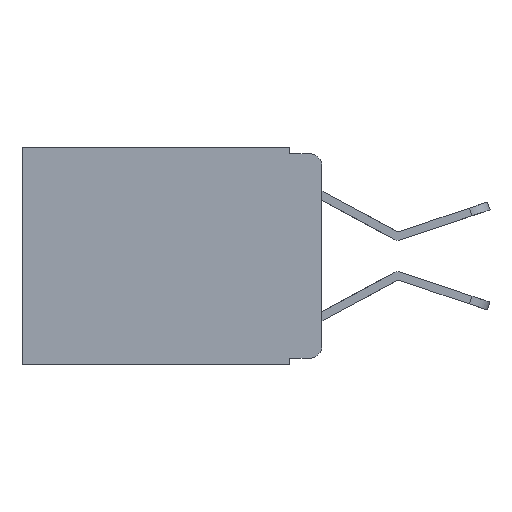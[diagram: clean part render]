
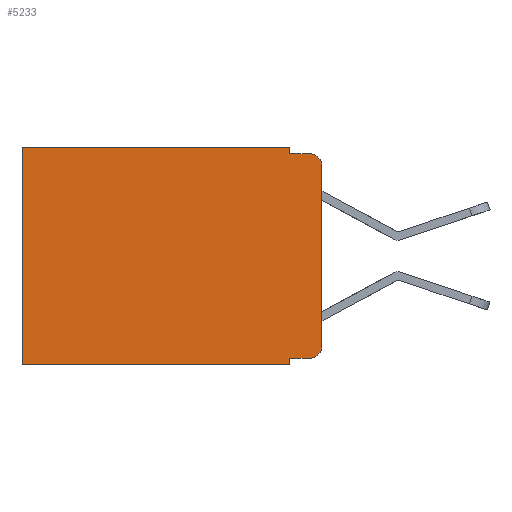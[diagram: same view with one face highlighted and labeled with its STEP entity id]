
A CAD part, left-side view. The second image highlights one B-rep face of the part: STEP entity #5233.
In plain terms, the highlighted planar face has unit normal (-1, 0, 0).
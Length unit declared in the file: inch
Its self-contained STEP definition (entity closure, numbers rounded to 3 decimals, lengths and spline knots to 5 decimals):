
#54 = CARTESIAN_POINT ( 'NONE',  ( 0.298, 0.473, -0.343 ) ) ;
#70 = PLANE ( 'NONE',  #1075 ) ;
#168 = VERTEX_POINT ( 'NONE', #1452 ) ;
#182 = DIRECTION ( 'NONE',  ( 0., 1., 0. ) ) ;
#252 = VERTEX_POINT ( 'NONE', #3909 ) ;
#328 = LINE ( 'NONE', #11626, #2485 ) ;
#396 = LINE ( 'NONE', #8816, #7727 ) ;
#457 = AXIS2_PLACEMENT_3D ( 'NONE', #2003, #8495, #3036 ) ;
#660 = DIRECTION ( 'NONE',  ( 0., 0., -1. ) ) ;
#685 = DIRECTION ( 'NONE',  ( 0., -1., 0. ) ) ;
#759 = CARTESIAN_POINT ( 'NONE',  ( 0.298, 0.051, -0.01 ) ) ;
#762 = ORIENTED_EDGE ( 'NONE', *, *, #2028, .F. ) ;
#1075 = AXIS2_PLACEMENT_3D ( 'NONE', #4985, #2177, #4659 ) ;
#1194 = CARTESIAN_POINT ( 'NONE',  ( 0.298, 0.051, -0.333 ) ) ;
#1288 = ORIENTED_EDGE ( 'NONE', *, *, #9350, .F. ) ;
#1316 = EDGE_LOOP ( 'NONE', ( #1550, #2362, #1288, #7834, #8016, #8745, #762, #8439, #8576, #10003 ) ) ;
#1383 = LINE ( 'NONE', #5748, #3727 ) ;
#1452 = CARTESIAN_POINT ( 'NONE',  ( 0.298, 0.02, -0.01 ) ) ;
#1543 = CARTESIAN_POINT ( 'NONE',  ( 0.298, 0.473, 0. ) ) ;
#1550 = ORIENTED_EDGE ( 'NONE', *, *, #5082, .F. ) ;
#1827 = DIRECTION ( 'NONE',  ( 0., -1., 0. ) ) ;
#1849 = CARTESIAN_POINT ( 'NONE',  ( 0.298, 0.051, -0.333 ) ) ;
#2003 = CARTESIAN_POINT ( 'NONE',  ( 0.298, 0.02, -0.03 ) ) ;
#2028 = EDGE_CURVE ( 'NONE', #7876, #8150, #396, .T. ) ;
#2152 = VERTEX_POINT ( 'NONE', #7052 ) ;
#2177 = DIRECTION ( 'NONE',  ( 1., 0., 0. ) ) ;
#2362 = ORIENTED_EDGE ( 'NONE', *, *, #11301, .T. ) ;
#2485 = VECTOR ( 'NONE', #660, 39.37008 ) ;
#2558 = VERTEX_POINT ( 'NONE', #5853 ) ;
#2632 = DIRECTION ( 'NONE',  ( -1., 0., 0. ) ) ;
#2672 = VECTOR ( 'NONE', #1827, 39.37008 ) ;
#2866 = VECTOR ( 'NONE', #10152, 39.37008 ) ;
#2903 = CARTESIAN_POINT ( 'NONE',  ( 0.298, 0., -0.03 ) ) ;
#2934 = EDGE_CURVE ( 'NONE', #6093, #2152, #1383, .T. ) ;
#2992 = LINE ( 'NONE', #8836, #7577 ) ;
#3036 = DIRECTION ( 'NONE',  ( 0., 0., -1. ) ) ;
#3727 = VECTOR ( 'NONE', #10771, 39.37008 ) ;
#3909 = CARTESIAN_POINT ( 'NONE',  ( 0.298, 0.02, -0.333 ) ) ;
#4335 = VECTOR ( 'NONE', #685, 39.37008 ) ;
#4659 = DIRECTION ( 'NONE',  ( 0., 0., -1. ) ) ;
#4985 = CARTESIAN_POINT ( 'NONE',  ( 0.298, 0., 0. ) ) ;
#5082 = EDGE_CURVE ( 'NONE', #10673, #2558, #11850, .T. ) ;
#5159 = EDGE_CURVE ( 'NONE', #7083, #252, #11622, .T. ) ;
#5176 = VERTEX_POINT ( 'NONE', #7269 ) ;
#5233 = ADVANCED_FACE ( 'NONE', ( #5897 ), #70, .F. ) ;
#5748 = CARTESIAN_POINT ( 'NONE',  ( 0.298, 0.051, 0. ) ) ;
#5853 = CARTESIAN_POINT ( 'NONE',  ( 0.298, 0., -0.313 ) ) ;
#5897 = FACE_OUTER_BOUND ( 'NONE', #1316, .T. ) ;
#6093 = VERTEX_POINT ( 'NONE', #7517 ) ;
#6402 = EDGE_CURVE ( 'NONE', #6093, #5176, #2992, .T. ) ;
#7052 = CARTESIAN_POINT ( 'NONE',  ( 0.298, 0.051, -0.01 ) ) ;
#7083 = VERTEX_POINT ( 'NONE', #1194 ) ;
#7269 = CARTESIAN_POINT ( 'NONE',  ( 0.298, 0.473, 0. ) ) ;
#7517 = CARTESIAN_POINT ( 'NONE',  ( 0.298, 0.051, 0. ) ) ;
#7566 = LINE ( 'NONE', #759, #2672 ) ;
#7577 = VECTOR ( 'NONE', #9701, 39.37008 ) ;
#7727 = VECTOR ( 'NONE', #182, 39.37008 ) ;
#7792 = CIRCLE ( 'NONE', #457, 0.02 ) ;
#7834 = ORIENTED_EDGE ( 'NONE', *, *, #2934, .F. ) ;
#7876 = VERTEX_POINT ( 'NONE', #10675 ) ;
#8016 = ORIENTED_EDGE ( 'NONE', *, *, #6402, .T. ) ;
#8104 = DIRECTION ( 'NONE',  ( 0., 0., -1. ) ) ;
#8139 = CARTESIAN_POINT ( 'NONE',  ( 0.298, 0.02, -0.313 ) ) ;
#8150 = VERTEX_POINT ( 'NONE', #54 ) ;
#8439 = ORIENTED_EDGE ( 'NONE', *, *, #10540, .F. ) ;
#8495 = DIRECTION ( 'NONE',  ( -1., 0., 0. ) ) ;
#8576 = ORIENTED_EDGE ( 'NONE', *, *, #5159, .T. ) ;
#8745 = ORIENTED_EDGE ( 'NONE', *, *, #11631, .T. ) ;
#8816 = CARTESIAN_POINT ( 'NONE',  ( 0.298, 0., -0.343 ) ) ;
#8836 = CARTESIAN_POINT ( 'NONE',  ( 0.298, 0., 0. ) ) ;
#9050 = DIRECTION ( 'NONE',  ( 0., 0., -1. ) ) ;
#9350 = EDGE_CURVE ( 'NONE', #2152, #168, #7566, .T. ) ;
#9701 = DIRECTION ( 'NONE',  ( 0., 1., 0. ) ) ;
#10003 = ORIENTED_EDGE ( 'NONE', *, *, #11090, .T. ) ;
#10152 = DIRECTION ( 'NONE',  ( 0., 0., -1. ) ) ;
#10306 = AXIS2_PLACEMENT_3D ( 'NONE', #8139, #2632, #9050 ) ;
#10392 = CARTESIAN_POINT ( 'NONE',  ( 0.298, 0., 0. ) ) ;
#10540 = EDGE_CURVE ( 'NONE', #7083, #7876, #328, .T. ) ;
#10659 = VECTOR ( 'NONE', #8104, 39.37008 ) ;
#10673 = VERTEX_POINT ( 'NONE', #2903 ) ;
#10675 = CARTESIAN_POINT ( 'NONE',  ( 0.298, 0.051, -0.343 ) ) ;
#10771 = DIRECTION ( 'NONE',  ( 0., 0., -1. ) ) ;
#10907 = LINE ( 'NONE', #1543, #10659 ) ;
#11090 = EDGE_CURVE ( 'NONE', #252, #2558, #11553, .T. ) ;
#11301 = EDGE_CURVE ( 'NONE', #10673, #168, #7792, .T. ) ;
#11553 = CIRCLE ( 'NONE', #10306, 0.02 ) ;
#11622 = LINE ( 'NONE', #1849, #4335 ) ;
#11626 = CARTESIAN_POINT ( 'NONE',  ( 0.298, 0.051, 0. ) ) ;
#11631 = EDGE_CURVE ( 'NONE', #5176, #8150, #10907, .T. ) ;
#11850 = LINE ( 'NONE', #10392, #2866 ) ;
